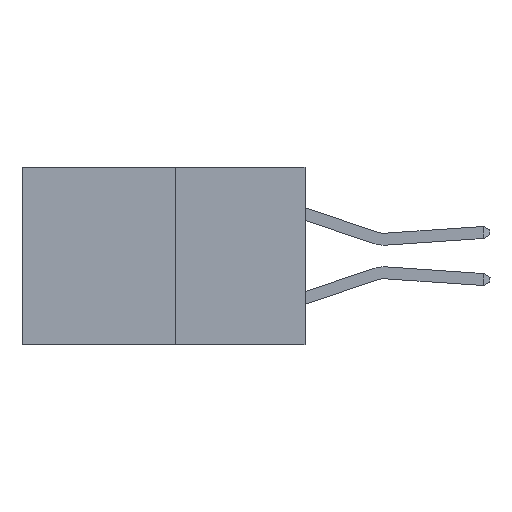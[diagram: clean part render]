
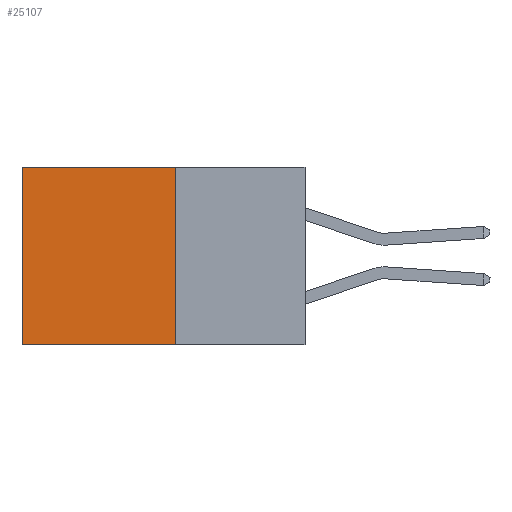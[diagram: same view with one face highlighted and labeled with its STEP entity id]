
A CAD part, left-side view. The second image highlights one B-rep face of the part: STEP entity #25107.
In plain terms, the highlighted planar face has unit normal (-1, 0, 0).
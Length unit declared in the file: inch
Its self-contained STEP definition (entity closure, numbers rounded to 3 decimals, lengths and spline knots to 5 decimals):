
#134 = DIRECTION ( 'NONE',  ( 1., 0., 0. ) ) ;
#182 = VECTOR ( 'NONE', #11669, 39.37008 ) ;
#221 = AXIS2_PLACEMENT_3D ( 'NONE', #7523, #134, #17492 ) ;
#259 = DIRECTION ( 'NONE',  ( 0., 0., -1. ) ) ;
#3272 = VERTEX_POINT ( 'NONE', #30272 ) ;
#3548 = EDGE_CURVE ( 'NONE', #10268, #9899, #4679, .T. ) ;
#4679 = LINE ( 'NONE', #21344, #23518 ) ;
#6454 = CARTESIAN_POINT ( 'NONE',  ( 0.277, 0.27, 0. ) ) ;
#6469 = EDGE_LOOP ( 'NONE', ( #12508, #10716, #26085, #27109 ) ) ;
#6556 = EDGE_CURVE ( 'NONE', #16582, #10268, #14161, .T. ) ;
#7130 = CARTESIAN_POINT ( 'NONE',  ( 0.277, 0.27, 0. ) ) ;
#7523 = CARTESIAN_POINT ( 'NONE',  ( 0.277, 0.27, -0.37 ) ) ;
#9899 = VERTEX_POINT ( 'NONE', #19173 ) ;
#10136 = VECTOR ( 'NONE', #259, 39.37008 ) ;
#10268 = VERTEX_POINT ( 'NONE', #14486 ) ;
#10716 = ORIENTED_EDGE ( 'NONE', *, *, #3548, .F. ) ;
#11493 = CARTESIAN_POINT ( 'NONE',  ( 0.277, 0.27, -0.37 ) ) ;
#11669 = DIRECTION ( 'NONE',  ( 0., 0., -1. ) ) ;
#12508 = ORIENTED_EDGE ( 'NONE', *, *, #27835, .T. ) ;
#14161 = LINE ( 'NONE', #11493, #182 ) ;
#14486 = CARTESIAN_POINT ( 'NONE',  ( 0.277, 0.27, -0.37 ) ) ;
#15001 = PLANE ( 'NONE',  #221 ) ;
#16533 = LINE ( 'NONE', #7130, #22233 ) ;
#16582 = VERTEX_POINT ( 'NONE', #6454 ) ;
#17096 = DIRECTION ( 'NONE',  ( 0., 1., 0. ) ) ;
#17492 = DIRECTION ( 'NONE',  ( 0., 0., -1. ) ) ;
#19173 = CARTESIAN_POINT ( 'NONE',  ( 0.277, 0.59, -0.37 ) ) ;
#21263 = DIRECTION ( 'NONE',  ( 0., 1., 0. ) ) ;
#21344 = CARTESIAN_POINT ( 'NONE',  ( 0.277, 0.27, -0.37 ) ) ;
#22233 = VECTOR ( 'NONE', #17096, 39.37008 ) ;
#23518 = VECTOR ( 'NONE', #21263, 39.37008 ) ;
#25107 = ADVANCED_FACE ( 'NONE', ( #28766 ), #15001, .F. ) ;
#26085 = ORIENTED_EDGE ( 'NONE', *, *, #6556, .F. ) ;
#26420 = EDGE_CURVE ( 'NONE', #16582, #3272, #16533, .T. ) ;
#27109 = ORIENTED_EDGE ( 'NONE', *, *, #26420, .T. ) ;
#27835 = EDGE_CURVE ( 'NONE', #3272, #9899, #29590, .T. ) ;
#28766 = FACE_OUTER_BOUND ( 'NONE', #6469, .T. ) ;
#29590 = LINE ( 'NONE', #29665, #10136 ) ;
#29665 = CARTESIAN_POINT ( 'NONE',  ( 0.277, 0.59, -0.37 ) ) ;
#30272 = CARTESIAN_POINT ( 'NONE',  ( 0.277, 0.59, 0. ) ) ;
